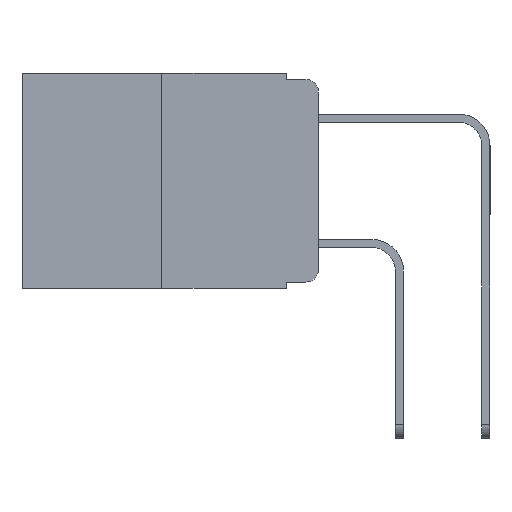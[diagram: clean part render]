
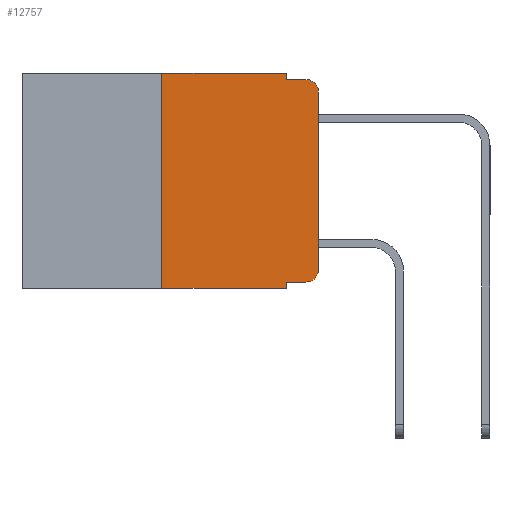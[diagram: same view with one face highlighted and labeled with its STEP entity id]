
A CAD part, left-side view. The second image highlights one B-rep face of the part: STEP entity #12757.
In plain terms, the highlighted planar face has unit normal (-1, 0, 0).
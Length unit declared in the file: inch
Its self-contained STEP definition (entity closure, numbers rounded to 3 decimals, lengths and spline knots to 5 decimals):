
#281 = DIRECTION ( 'NONE',  ( 0., 0., -1. ) ) ;
#309 = ORIENTED_EDGE ( 'NONE', *, *, #11931, .T. ) ;
#614 = VECTOR ( 'NONE', #1315, 39.37008 ) ;
#673 = VERTEX_POINT ( 'NONE', #1184 ) ;
#695 = ORIENTED_EDGE ( 'NONE', *, *, #13536, .F. ) ;
#815 = DIRECTION ( 'NONE',  ( -1., 0., 0. ) ) ;
#1025 = DIRECTION ( 'NONE',  ( 1., 0., 0. ) ) ;
#1159 = ORIENTED_EDGE ( 'NONE', *, *, #9864, .F. ) ;
#1184 = CARTESIAN_POINT ( 'NONE',  ( 0., 0.051, -0.343 ) ) ;
#1306 = CARTESIAN_POINT ( 'NONE',  ( 0., 0.051, -0.01 ) ) ;
#1315 = DIRECTION ( 'NONE',  ( 0., -1., 0. ) ) ;
#1448 = VERTEX_POINT ( 'NONE', #13421 ) ;
#1810 = ORIENTED_EDGE ( 'NONE', *, *, #13000, .T. ) ;
#2060 = PLANE ( 'NONE',  #10690 ) ;
#2137 = CARTESIAN_POINT ( 'NONE',  ( 0., 0.25, 0. ) ) ;
#2389 = CARTESIAN_POINT ( 'NONE',  ( 0., 0.02, -0.313 ) ) ;
#2472 = LINE ( 'NONE', #11999, #4967 ) ;
#2555 = ORIENTED_EDGE ( 'NONE', *, *, #10000, .T. ) ;
#3008 = LINE ( 'NONE', #3770, #5544 ) ;
#3395 = VERTEX_POINT ( 'NONE', #10853 ) ;
#3408 = VECTOR ( 'NONE', #6679, 39.37008 ) ;
#3438 = DIRECTION ( 'NONE',  ( 0., 0., -1. ) ) ;
#3451 = LINE ( 'NONE', #4458, #614 ) ;
#3528 = EDGE_LOOP ( 'NONE', ( #5503, #309, #4925, #1159, #695, #6228, #1810, #3805, #2555, #4314 ) ) ;
#3573 = VERTEX_POINT ( 'NONE', #5923 ) ;
#3770 = CARTESIAN_POINT ( 'NONE',  ( 0., 0.473, -0.343 ) ) ;
#3805 = ORIENTED_EDGE ( 'NONE', *, *, #4972, .F. ) ;
#4314 = ORIENTED_EDGE ( 'NONE', *, *, #5273, .T. ) ;
#4355 = CIRCLE ( 'NONE', #4804, 0.02 ) ;
#4458 = CARTESIAN_POINT ( 'NONE',  ( 0., 0.051, -0.01 ) ) ;
#4740 = VECTOR ( 'NONE', #8495, 39.37008 ) ;
#4804 = AXIS2_PLACEMENT_3D ( 'NONE', #2389, #9812, #3438 ) ;
#4925 = ORIENTED_EDGE ( 'NONE', *, *, #13434, .F. ) ;
#4967 = VECTOR ( 'NONE', #8820, 39.37008 ) ;
#4972 = EDGE_CURVE ( 'NONE', #3573, #673, #5210, .T. ) ;
#5210 = LINE ( 'NONE', #7027, #13262 ) ;
#5273 = EDGE_CURVE ( 'NONE', #12709, #6545, #4355, .T. ) ;
#5503 = ORIENTED_EDGE ( 'NONE', *, *, #11450, .T. ) ;
#5544 = VECTOR ( 'NONE', #11182, 39.37008 ) ;
#5923 = CARTESIAN_POINT ( 'NONE',  ( 0., 0.051, -0.333 ) ) ;
#6228 = ORIENTED_EDGE ( 'NONE', *, *, #8533, .F. ) ;
#6257 = LINE ( 'NONE', #6634, #3408 ) ;
#6299 = CARTESIAN_POINT ( 'NONE',  ( 0., 0.02, -0.333 ) ) ;
#6303 = LINE ( 'NONE', #2137, #11583 ) ;
#6545 = VERTEX_POINT ( 'NONE', #12969 ) ;
#6634 = CARTESIAN_POINT ( 'NONE',  ( 0., 0.051, 0. ) ) ;
#6679 = DIRECTION ( 'NONE',  ( 0., 0., -1. ) ) ;
#6895 = VERTEX_POINT ( 'NONE', #12518 ) ;
#7027 = CARTESIAN_POINT ( 'NONE',  ( 0., 0.051, 0. ) ) ;
#7190 = CARTESIAN_POINT ( 'NONE',  ( 0., 0.02, -0.03 ) ) ;
#7400 = CARTESIAN_POINT ( 'NONE',  ( 0., 0.473, 0. ) ) ;
#7436 = CARTESIAN_POINT ( 'NONE',  ( 0., 0., 0. ) ) ;
#8073 = VECTOR ( 'NONE', #13117, 39.37008 ) ;
#8251 = DIRECTION ( 'NONE',  ( 0., 0., -1. ) ) ;
#8469 = DIRECTION ( 'NONE',  ( 0., 0., -1. ) ) ;
#8495 = DIRECTION ( 'NONE',  ( 0., 0., 1. ) ) ;
#8516 = FACE_OUTER_BOUND ( 'NONE', #3528, .T. ) ;
#8533 = EDGE_CURVE ( 'NONE', #1448, #8922, #6303, .T. ) ;
#8591 = DIRECTION ( 'NONE',  ( 0., 0., 1. ) ) ;
#8820 = DIRECTION ( 'NONE',  ( 0., -1., 0. ) ) ;
#8922 = VERTEX_POINT ( 'NONE', #10284 ) ;
#9328 = CARTESIAN_POINT ( 'NONE',  ( 0., 0., -0.03 ) ) ;
#9812 = DIRECTION ( 'NONE',  ( -1., 0., 0. ) ) ;
#9864 = EDGE_CURVE ( 'NONE', #3395, #10548, #6257, .T. ) ;
#10000 = EDGE_CURVE ( 'NONE', #3573, #12709, #12992, .T. ) ;
#10284 = CARTESIAN_POINT ( 'NONE',  ( 0., 0.25, 0. ) ) ;
#10548 = VERTEX_POINT ( 'NONE', #1306 ) ;
#10690 = AXIS2_PLACEMENT_3D ( 'NONE', #7400, #1025, #8469 ) ;
#10853 = CARTESIAN_POINT ( 'NONE',  ( 0., 0.051, 0. ) ) ;
#11089 = CARTESIAN_POINT ( 'NONE',  ( 0., 0.051, -0.333 ) ) ;
#11182 = DIRECTION ( 'NONE',  ( 0., -1., 0. ) ) ;
#11328 = VERTEX_POINT ( 'NONE', #9328 ) ;
#11450 = EDGE_CURVE ( 'NONE', #6545, #11328, #13441, .T. ) ;
#11583 = VECTOR ( 'NONE', #8591, 39.37008 ) ;
#11931 = EDGE_CURVE ( 'NONE', #11328, #6895, #12483, .T. ) ;
#11999 = CARTESIAN_POINT ( 'NONE',  ( 0., 0.473, 0. ) ) ;
#12174 = AXIS2_PLACEMENT_3D ( 'NONE', #7190, #815, #8251 ) ;
#12483 = CIRCLE ( 'NONE', #12174, 0.02 ) ;
#12518 = CARTESIAN_POINT ( 'NONE',  ( 0., 0.02, -0.01 ) ) ;
#12709 = VERTEX_POINT ( 'NONE', #6299 ) ;
#12757 = ADVANCED_FACE ( 'NONE', ( #8516 ), #2060, .F. ) ;
#12969 = CARTESIAN_POINT ( 'NONE',  ( 0., 0., -0.313 ) ) ;
#12992 = LINE ( 'NONE', #11089, #8073 ) ;
#13000 = EDGE_CURVE ( 'NONE', #1448, #673, #3008, .T. ) ;
#13117 = DIRECTION ( 'NONE',  ( 0., -1., 0. ) ) ;
#13262 = VECTOR ( 'NONE', #281, 39.37008 ) ;
#13421 = CARTESIAN_POINT ( 'NONE',  ( 0., 0.25, -0.343 ) ) ;
#13434 = EDGE_CURVE ( 'NONE', #10548, #6895, #3451, .T. ) ;
#13441 = LINE ( 'NONE', #7436, #4740 ) ;
#13536 = EDGE_CURVE ( 'NONE', #8922, #3395, #2472, .T. ) ;
